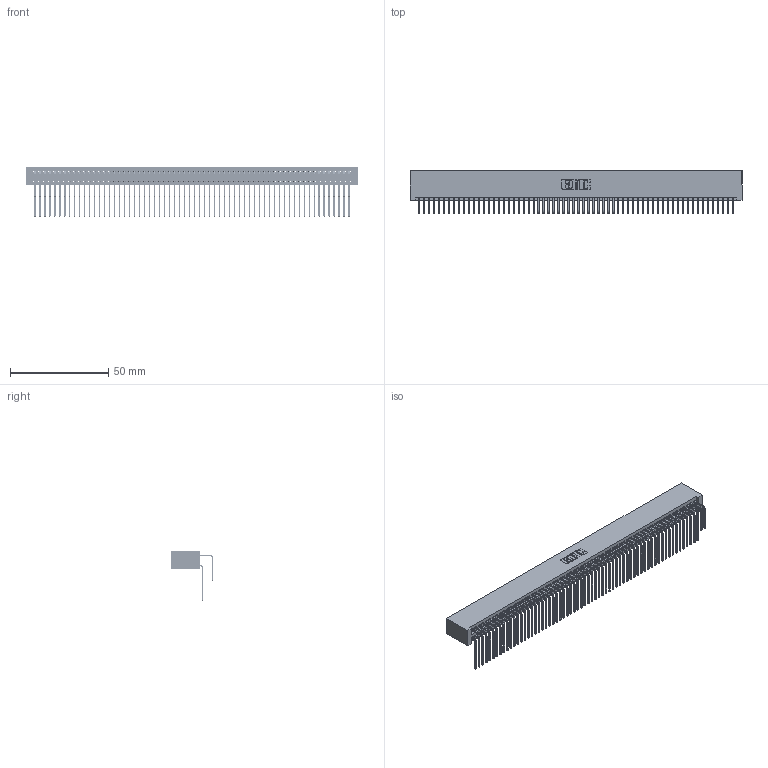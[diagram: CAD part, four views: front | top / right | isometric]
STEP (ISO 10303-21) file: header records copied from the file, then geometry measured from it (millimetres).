
FILE_DESCRIPTION (( 'STEP AP203' ), '1' );
FILE_NAME ('395-128-558-201.STEP', '2018-12-04T13:26:51', ( '' ), ( '' ), 'SwSTEP 2.0', 'SolidWorks 2016', '' );
FILE_SCHEMA (( 'CONFIG_CONTROL_DESIGN' ));
Length unit declared in the file: inch
Products named in the file (4): 395-128-558-201; 345 Part_No Mounting Lugs; 345-292-001_558 Tail - 2; 345-292-001_558 559 Tail - 1
Assembly tree (129 placements, depth 2):
  395-128-558-201
    345 Part_No Mounting Lugs
    345-292-001_558 559 Tail - 1  x64
    345-292-001_558 Tail - 2  x64
Bounding box: 169.16 x 21.83 x 25.53 mm (x, y, z)
Volume: 17991.3 mm3; surface area: 30795.7 mm2
Topology: 129 solids, 129 shells, 6774 faces, 20157 edges, 13266 vertices
Faces by surface type: plane 4556, cylinder 2218
Entity records: 48629 total; most frequent: CARTESIAN_POINT 8175, ORIENTED_EDGE 8058, DIRECTION 7149, EDGE_CURVE 4029, LINE 3609, VECTOR 3609, VERTEX_POINT 2682, AXIS2_PLACEMENT_3D 1770
